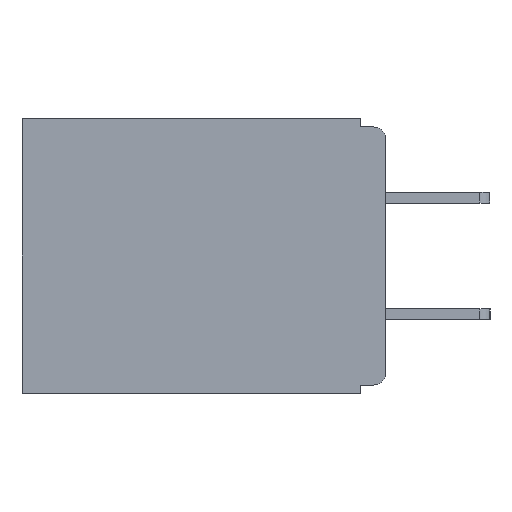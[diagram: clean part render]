
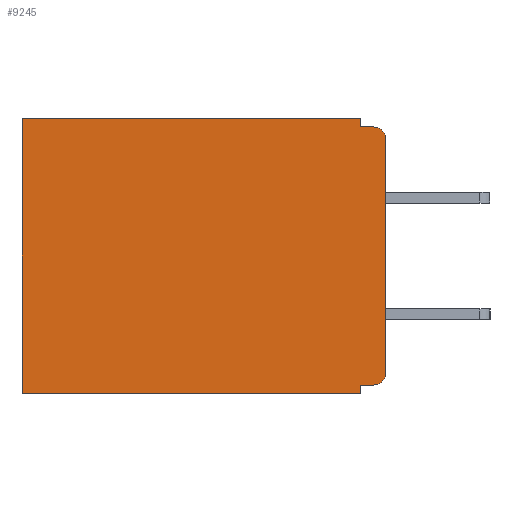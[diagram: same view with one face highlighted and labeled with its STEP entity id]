
A CAD part, left-side view. The second image highlights one B-rep face of the part: STEP entity #9245.
In plain terms, the highlighted planar face has unit normal (-1, 0, 0).
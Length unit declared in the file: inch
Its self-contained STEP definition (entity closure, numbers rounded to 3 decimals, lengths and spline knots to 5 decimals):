
#137 = CARTESIAN_POINT ( 'NONE',  ( 0.3, 0., 0. ) ) ;
#173 = VECTOR ( 'NONE', #7278, 39.37008 ) ;
#180 = EDGE_LOOP ( 'NONE', ( #10532, #539, #8352, #10945, #4903, #7526, #7512, #6172, #3623, #5113 ) ) ;
#531 = CARTESIAN_POINT ( 'NONE',  ( 0.3, 0.031, -0.32 ) ) ;
#539 = ORIENTED_EDGE ( 'NONE', *, *, #6515, .T. ) ;
#990 = AXIS2_PLACEMENT_3D ( 'NONE', #11990, #12103, #11742 ) ;
#1134 = LINE ( 'NONE', #6523, #13197 ) ;
#1168 = EDGE_CURVE ( 'NONE', #5058, #14003, #12544, .T. ) ;
#1581 = CARTESIAN_POINT ( 'NONE',  ( 0.3, 0.015, -0.32 ) ) ;
#1766 = LINE ( 'NONE', #5899, #2477 ) ;
#2477 = VECTOR ( 'NONE', #14239, 39.37008 ) ;
#2637 = VERTEX_POINT ( 'NONE', #4097 ) ;
#2672 = VERTEX_POINT ( 'NONE', #4639 ) ;
#3168 = EDGE_CURVE ( 'NONE', #7736, #2672, #1766, .T. ) ;
#3171 = VECTOR ( 'NONE', #14784, 39.37008 ) ;
#3211 = CARTESIAN_POINT ( 'NONE',  ( 0.3, 0., -0.32 ) ) ;
#3623 = ORIENTED_EDGE ( 'NONE', *, *, #1168, .F. ) ;
#3827 = CIRCLE ( 'NONE', #13329, 0.015 ) ;
#4097 = CARTESIAN_POINT ( 'NONE',  ( 0.3, 0.015, -0.01 ) ) ;
#4224 = EDGE_CURVE ( 'NONE', #10317, #9005, #10953, .T. ) ;
#4328 = EDGE_CURVE ( 'NONE', #12106, #2637, #6422, .T. ) ;
#4639 = CARTESIAN_POINT ( 'NONE',  ( 0.3, 0., -0.305 ) ) ;
#4653 = CIRCLE ( 'NONE', #990, 0.015 ) ;
#4696 = AXIS2_PLACEMENT_3D ( 'NONE', #7057, #6997, #6982 ) ;
#4822 = LINE ( 'NONE', #10219, #11044 ) ;
#4903 = ORIENTED_EDGE ( 'NONE', *, *, #11438, .T. ) ;
#5058 = VERTEX_POINT ( 'NONE', #1581 ) ;
#5096 = FACE_OUTER_BOUND ( 'NONE', #180, .T. ) ;
#5113 = ORIENTED_EDGE ( 'NONE', *, *, #8644, .T. ) ;
#5899 = CARTESIAN_POINT ( 'NONE',  ( 0.3, 0., -0.33 ) ) ;
#6108 = EDGE_CURVE ( 'NONE', #14230, #12106, #1134, .T. ) ;
#6172 = ORIENTED_EDGE ( 'NONE', *, *, #11799, .F. ) ;
#6422 = LINE ( 'NONE', #14993, #3171 ) ;
#6515 = EDGE_CURVE ( 'NONE', #7736, #2637, #4653, .T. ) ;
#6520 = LINE ( 'NONE', #137, #173 ) ;
#6523 = CARTESIAN_POINT ( 'NONE',  ( 0.3, 0.031, 0. ) ) ;
#6539 = DIRECTION ( 'NONE',  ( 0., 0., -1. ) ) ;
#6586 = CARTESIAN_POINT ( 'NONE',  ( 0.3, 0.437, -0.33 ) ) ;
#6982 = DIRECTION ( 'NONE',  ( 0., 0., -1. ) ) ;
#6997 = DIRECTION ( 'NONE',  ( 1., 0., 0. ) ) ;
#7057 = CARTESIAN_POINT ( 'NONE',  ( 0.3, 0., -0.33 ) ) ;
#7130 = PLANE ( 'NONE',  #4696 ) ;
#7278 = DIRECTION ( 'NONE',  ( 0., 1., 0. ) ) ;
#7507 = LINE ( 'NONE', #6586, #13237 ) ;
#7512 = ORIENTED_EDGE ( 'NONE', *, *, #4224, .F. ) ;
#7526 = ORIENTED_EDGE ( 'NONE', *, *, #9314, .T. ) ;
#7715 = DIRECTION ( 'NONE',  ( 0., 1., 0. ) ) ;
#7736 = VERTEX_POINT ( 'NONE', #8459 ) ;
#8352 = ORIENTED_EDGE ( 'NONE', *, *, #4328, .F. ) ;
#8459 = CARTESIAN_POINT ( 'NONE',  ( 0.3, 0., -0.025 ) ) ;
#8644 = EDGE_CURVE ( 'NONE', #5058, #2672, #3827, .T. ) ;
#8800 = CARTESIAN_POINT ( 'NONE',  ( 0.3, 0.437, 0. ) ) ;
#8804 = CARTESIAN_POINT ( 'NONE',  ( 0.3, 0.031, -0.33 ) ) ;
#9005 = VERTEX_POINT ( 'NONE', #9174 ) ;
#9174 = CARTESIAN_POINT ( 'NONE',  ( 0.3, 0.437, -0.33 ) ) ;
#9245 = ADVANCED_FACE ( 'NONE', ( #5096 ), #7130, .F. ) ;
#9314 = EDGE_CURVE ( 'NONE', #13959, #9005, #7507, .T. ) ;
#9501 = VECTOR ( 'NONE', #7715, 39.37008 ) ;
#10219 = CARTESIAN_POINT ( 'NONE',  ( 0.3, 0.031, -0.33 ) ) ;
#10317 = VERTEX_POINT ( 'NONE', #8804 ) ;
#10532 = ORIENTED_EDGE ( 'NONE', *, *, #3168, .F. ) ;
#10791 = CARTESIAN_POINT ( 'NONE',  ( 0.3, 0., -0.33 ) ) ;
#10945 = ORIENTED_EDGE ( 'NONE', *, *, #6108, .F. ) ;
#10953 = LINE ( 'NONE', #10791, #13585 ) ;
#11044 = VECTOR ( 'NONE', #13642, 39.37008 ) ;
#11153 = DIRECTION ( 'NONE',  ( 0., 1., 0. ) ) ;
#11438 = EDGE_CURVE ( 'NONE', #14230, #13959, #6520, .T. ) ;
#11655 = DIRECTION ( 'NONE',  ( 0., 0., -1. ) ) ;
#11664 = DIRECTION ( 'NONE',  ( -1., 0., 0. ) ) ;
#11668 = CARTESIAN_POINT ( 'NONE',  ( 0.3, 0.015, -0.305 ) ) ;
#11742 = DIRECTION ( 'NONE',  ( 0., 0., -1. ) ) ;
#11799 = EDGE_CURVE ( 'NONE', #14003, #10317, #4822, .T. ) ;
#11910 = CARTESIAN_POINT ( 'NONE',  ( 0.3, 0.031, -0.01 ) ) ;
#11990 = CARTESIAN_POINT ( 'NONE',  ( 0.3, 0.015, -0.025 ) ) ;
#12042 = DIRECTION ( 'NONE',  ( 0., 0., -1. ) ) ;
#12103 = DIRECTION ( 'NONE',  ( -1., 0., 0. ) ) ;
#12106 = VERTEX_POINT ( 'NONE', #11910 ) ;
#12544 = LINE ( 'NONE', #3211, #9501 ) ;
#13197 = VECTOR ( 'NONE', #12042, 39.37008 ) ;
#13237 = VECTOR ( 'NONE', #6539, 39.37008 ) ;
#13329 = AXIS2_PLACEMENT_3D ( 'NONE', #11668, #11664, #11655 ) ;
#13585 = VECTOR ( 'NONE', #11153, 39.37008 ) ;
#13642 = DIRECTION ( 'NONE',  ( 0., 0., -1. ) ) ;
#13762 = CARTESIAN_POINT ( 'NONE',  ( 0.3, 0.031, 0. ) ) ;
#13959 = VERTEX_POINT ( 'NONE', #8800 ) ;
#14003 = VERTEX_POINT ( 'NONE', #531 ) ;
#14230 = VERTEX_POINT ( 'NONE', #13762 ) ;
#14239 = DIRECTION ( 'NONE',  ( 0., 0., -1. ) ) ;
#14784 = DIRECTION ( 'NONE',  ( 0., -1., 0. ) ) ;
#14993 = CARTESIAN_POINT ( 'NONE',  ( 0.3, 0., -0.01 ) ) ;
